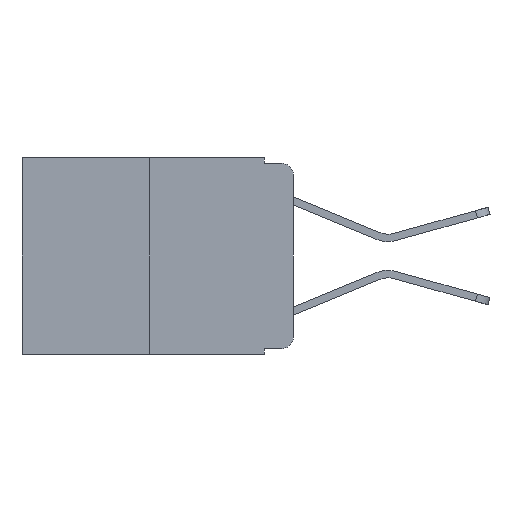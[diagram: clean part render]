
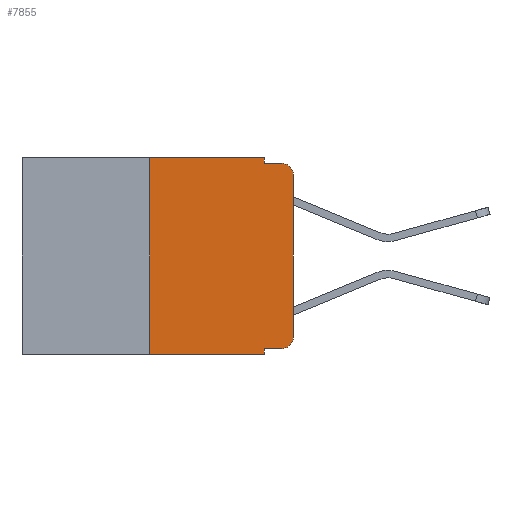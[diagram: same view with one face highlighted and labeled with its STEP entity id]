
A CAD part, left-side view. The second image highlights one B-rep face of the part: STEP entity #7855.
In plain terms, the highlighted planar face has unit normal (-1, 0, 0).
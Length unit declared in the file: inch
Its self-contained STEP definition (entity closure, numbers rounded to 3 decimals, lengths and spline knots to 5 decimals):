
#45 = VERTEX_POINT ( 'NONE', #19009 ) ;
#161 = DIRECTION ( 'NONE',  ( 0., 0., 1. ) ) ;
#163 = ORIENTED_EDGE ( 'NONE', *, *, #12172, .T. ) ;
#398 = VECTOR ( 'NONE', #14521, 39.37008 ) ;
#865 = CARTESIAN_POINT ( 'NONE',  ( 0., 0.051, -0.01 ) ) ;
#911 = CARTESIAN_POINT ( 'NONE',  ( 0., 0.051, -0.333 ) ) ;
#1553 = CARTESIAN_POINT ( 'NONE',  ( 0., 0.25, -0.343 ) ) ;
#1570 = ORIENTED_EDGE ( 'NONE', *, *, #10576, .T. ) ;
#2162 = LINE ( 'NONE', #8603, #13641 ) ;
#2198 = EDGE_CURVE ( 'NONE', #19241, #18241, #8851, .T. ) ;
#2639 = ORIENTED_EDGE ( 'NONE', *, *, #14976, .F. ) ;
#2697 = DIRECTION ( 'NONE',  ( 0., -1., 0. ) ) ;
#3030 = EDGE_CURVE ( 'NONE', #45, #6716, #8838, .T. ) ;
#3238 = CARTESIAN_POINT ( 'NONE',  ( 0., 0.051, 0. ) ) ;
#3300 = DIRECTION ( 'NONE',  ( 1., 0., 0. ) ) ;
#3369 = VERTEX_POINT ( 'NONE', #4436 ) ;
#3636 = EDGE_LOOP ( 'NONE', ( #14100, #9886, #9831, #2639, #11637, #8867, #1570, #17064, #163, #13399 ) ) ;
#3732 = EDGE_CURVE ( 'NONE', #17959, #3369, #5275, .T. ) ;
#3971 = VECTOR ( 'NONE', #20245, 39.37008 ) ;
#4161 = EDGE_CURVE ( 'NONE', #11750, #19241, #16977, .T. ) ;
#4436 = CARTESIAN_POINT ( 'NONE',  ( 0., 0.02, -0.01 ) ) ;
#4901 = EDGE_CURVE ( 'NONE', #5527, #3369, #12755, .T. ) ;
#5049 = LINE ( 'NONE', #14455, #398 ) ;
#5220 = CARTESIAN_POINT ( 'NONE',  ( 0., 0.25, 0. ) ) ;
#5275 = LINE ( 'NONE', #865, #17487 ) ;
#5527 = VERTEX_POINT ( 'NONE', #9877 ) ;
#5864 = CARTESIAN_POINT ( 'NONE',  ( 0., 0.051, 0. ) ) ;
#6211 = FACE_OUTER_BOUND ( 'NONE', #3636, .T. ) ;
#6716 = VERTEX_POINT ( 'NONE', #10673 ) ;
#7288 = CARTESIAN_POINT ( 'NONE',  ( 0., 0.02, -0.313 ) ) ;
#7398 = VECTOR ( 'NONE', #2697, 39.37008 ) ;
#7464 = CARTESIAN_POINT ( 'NONE',  ( 0., 0.25, 0. ) ) ;
#7736 = VERTEX_POINT ( 'NONE', #15885 ) ;
#7855 = ADVANCED_FACE ( 'NONE', ( #6211 ), #8246, .F. ) ;
#8246 = PLANE ( 'NONE',  #17357 ) ;
#8296 = LINE ( 'NONE', #5864, #20315 ) ;
#8603 = CARTESIAN_POINT ( 'NONE',  ( 0., 0., 0. ) ) ;
#8838 = LINE ( 'NONE', #20011, #20852 ) ;
#8851 = LINE ( 'NONE', #16477, #3971 ) ;
#8867 = ORIENTED_EDGE ( 'NONE', *, *, #4161, .F. ) ;
#8885 = DIRECTION ( 'NONE',  ( 0., 0., -1. ) ) ;
#9239 = EDGE_CURVE ( 'NONE', #17738, #5527, #2162, .T. ) ;
#9831 = ORIENTED_EDGE ( 'NONE', *, *, #3732, .F. ) ;
#9877 = CARTESIAN_POINT ( 'NONE',  ( 0., 0., -0.03 ) ) ;
#9886 = ORIENTED_EDGE ( 'NONE', *, *, #4901, .T. ) ;
#10576 = EDGE_CURVE ( 'NONE', #11750, #6716, #5049, .T. ) ;
#10673 = CARTESIAN_POINT ( 'NONE',  ( 0., 0.051, -0.343 ) ) ;
#11637 = ORIENTED_EDGE ( 'NONE', *, *, #2198, .F. ) ;
#11750 = VERTEX_POINT ( 'NONE', #1553 ) ;
#11907 = DIRECTION ( 'NONE',  ( -1., 0., 0. ) ) ;
#12172 = EDGE_CURVE ( 'NONE', #45, #7736, #15867, .T. ) ;
#12446 = DIRECTION ( 'NONE',  ( 0., 0., 1. ) ) ;
#12755 = CIRCLE ( 'NONE', #14970, 0.02 ) ;
#12789 = VECTOR ( 'NONE', #12446, 39.37008 ) ;
#13032 = CARTESIAN_POINT ( 'NONE',  ( 0., 0.473, 0. ) ) ;
#13399 = ORIENTED_EDGE ( 'NONE', *, *, #17821, .T. ) ;
#13641 = VECTOR ( 'NONE', #161, 39.37008 ) ;
#14100 = ORIENTED_EDGE ( 'NONE', *, *, #9239, .T. ) ;
#14455 = CARTESIAN_POINT ( 'NONE',  ( 0., 0.473, -0.343 ) ) ;
#14464 = CARTESIAN_POINT ( 'NONE',  ( 0., 0.02, -0.03 ) ) ;
#14521 = DIRECTION ( 'NONE',  ( 0., -1., 0. ) ) ;
#14620 = DIRECTION ( 'NONE',  ( 0., 0., -1. ) ) ;
#14970 = AXIS2_PLACEMENT_3D ( 'NONE', #14464, #11907, #20025 ) ;
#14976 = EDGE_CURVE ( 'NONE', #18241, #17959, #8296, .T. ) ;
#15489 = DIRECTION ( 'NONE',  ( 0., 0., -1. ) ) ;
#15867 = LINE ( 'NONE', #911, #7398 ) ;
#15885 = CARTESIAN_POINT ( 'NONE',  ( 0., 0.02, -0.333 ) ) ;
#16477 = CARTESIAN_POINT ( 'NONE',  ( 0., 0.473, 0. ) ) ;
#16977 = LINE ( 'NONE', #5220, #12789 ) ;
#17064 = ORIENTED_EDGE ( 'NONE', *, *, #3030, .F. ) ;
#17128 = CARTESIAN_POINT ( 'NONE',  ( 0., 0.051, -0.01 ) ) ;
#17357 = AXIS2_PLACEMENT_3D ( 'NONE', #13032, #3300, #14620 ) ;
#17487 = VECTOR ( 'NONE', #17906, 39.37008 ) ;
#17738 = VERTEX_POINT ( 'NONE', #17796 ) ;
#17796 = CARTESIAN_POINT ( 'NONE',  ( 0., 0., -0.313 ) ) ;
#17821 = EDGE_CURVE ( 'NONE', #7736, #17738, #20944, .T. ) ;
#17906 = DIRECTION ( 'NONE',  ( 0., -1., 0. ) ) ;
#17959 = VERTEX_POINT ( 'NONE', #17128 ) ;
#18241 = VERTEX_POINT ( 'NONE', #3238 ) ;
#18317 = DIRECTION ( 'NONE',  ( -1., 0., 0. ) ) ;
#18523 = AXIS2_PLACEMENT_3D ( 'NONE', #7288, #18317, #8885 ) ;
#19009 = CARTESIAN_POINT ( 'NONE',  ( 0., 0.051, -0.333 ) ) ;
#19241 = VERTEX_POINT ( 'NONE', #7464 ) ;
#19918 = DIRECTION ( 'NONE',  ( 0., 0., -1. ) ) ;
#20011 = CARTESIAN_POINT ( 'NONE',  ( 0., 0.051, 0. ) ) ;
#20025 = DIRECTION ( 'NONE',  ( 0., 0., -1. ) ) ;
#20245 = DIRECTION ( 'NONE',  ( 0., -1., 0. ) ) ;
#20315 = VECTOR ( 'NONE', #15489, 39.37008 ) ;
#20852 = VECTOR ( 'NONE', #19918, 39.37008 ) ;
#20944 = CIRCLE ( 'NONE', #18523, 0.02 ) ;
